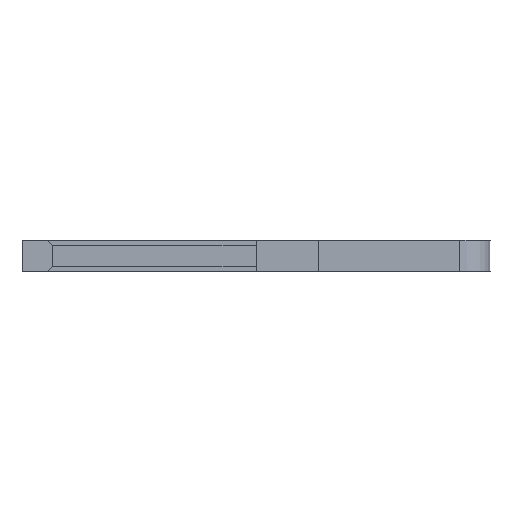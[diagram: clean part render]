
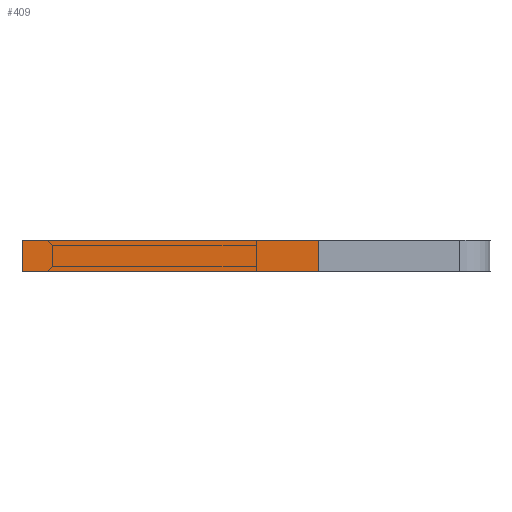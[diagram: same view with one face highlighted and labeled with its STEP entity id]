
A CAD part, left-side view. The second image highlights one B-rep face of the part: STEP entity #409.
In plain terms, the highlighted face is planar.
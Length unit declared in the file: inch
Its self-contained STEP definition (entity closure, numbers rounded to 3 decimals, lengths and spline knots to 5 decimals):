
#27 = CARTESIAN_POINT ( 'NONE',  ( -0.01, 0.15, -0.04 ) ) ;
#152 = CARTESIAN_POINT ( 'NONE',  ( -0.01, -0.04, -0.04 ) ) ;
#259 = CARTESIAN_POINT ( 'NONE',  ( 0.01, 0.15, -0.04 ) ) ;
#409 = ADVANCED_FACE ( 'NONE', ( #1319 ), #2372, .F. ) ;
#653 = VERTEX_POINT ( 'NONE', #1749 ) ;
#802 = VECTOR ( 'NONE', #1858, 39.37008 ) ;
#938 = ORIENTED_EDGE ( 'NONE', *, *, #4254, .F. ) ;
#1319 = FACE_OUTER_BOUND ( 'NONE', #3936, .T. ) ;
#1463 = LINE ( 'NONE', #2162, #802 ) ;
#1688 = CARTESIAN_POINT ( 'NONE',  ( 0.01, 0.15, -0.04 ) ) ;
#1713 = DIRECTION ( 'NONE',  ( 0., 1., 0. ) ) ;
#1749 = CARTESIAN_POINT ( 'NONE',  ( 0.01, 0.15, -0.04 ) ) ;
#1798 = CARTESIAN_POINT ( 'NONE',  ( -0.01, 0.15, -0.04 ) ) ;
#1858 = DIRECTION ( 'NONE',  ( -1., 0., 0. ) ) ;
#1868 = EDGE_CURVE ( 'NONE', #2222, #2746, #2021, .T. ) ;
#1905 = VECTOR ( 'NONE', #2561, 39.37008 ) ;
#1966 = EDGE_CURVE ( 'NONE', #4165, #2222, #1463, .T. ) ;
#2021 = LINE ( 'NONE', #1798, #1905 ) ;
#2094 = CARTESIAN_POINT ( 'NONE',  ( 0.01, -0.04, -0.04 ) ) ;
#2162 = CARTESIAN_POINT ( 'NONE',  ( 0.01, -0.04, -0.04 ) ) ;
#2198 = LINE ( 'NONE', #3051, #2648 ) ;
#2222 = VERTEX_POINT ( 'NONE', #152 ) ;
#2372 = PLANE ( 'NONE',  #3768 ) ;
#2561 = DIRECTION ( 'NONE',  ( 0., 1., 0. ) ) ;
#2648 = VECTOR ( 'NONE', #2677, 39.37008 ) ;
#2677 = DIRECTION ( 'NONE',  ( -1., 0., 0. ) ) ;
#2746 = VERTEX_POINT ( 'NONE', #27 ) ;
#2764 = DIRECTION ( 'NONE',  ( 0., 0., 1. ) ) ;
#3051 = CARTESIAN_POINT ( 'NONE',  ( 0.01, 0.15, -0.04 ) ) ;
#3279 = EDGE_CURVE ( 'NONE', #653, #2746, #2198, .T. ) ;
#3364 = ORIENTED_EDGE ( 'NONE', *, *, #1966, .T. ) ;
#3502 = DIRECTION ( 'NONE',  ( 1., 0., 0. ) ) ;
#3629 = VECTOR ( 'NONE', #1713, 39.37008 ) ;
#3662 = ORIENTED_EDGE ( 'NONE', *, *, #1868, .T. ) ;
#3768 = AXIS2_PLACEMENT_3D ( 'NONE', #1688, #2764, #3502 ) ;
#3936 = EDGE_LOOP ( 'NONE', ( #3662, #4031, #938, #3364 ) ) ;
#4031 = ORIENTED_EDGE ( 'NONE', *, *, #3279, .F. ) ;
#4079 = LINE ( 'NONE', #259, #3629 ) ;
#4165 = VERTEX_POINT ( 'NONE', #2094 ) ;
#4254 = EDGE_CURVE ( 'NONE', #4165, #653, #4079, .T. ) ;
